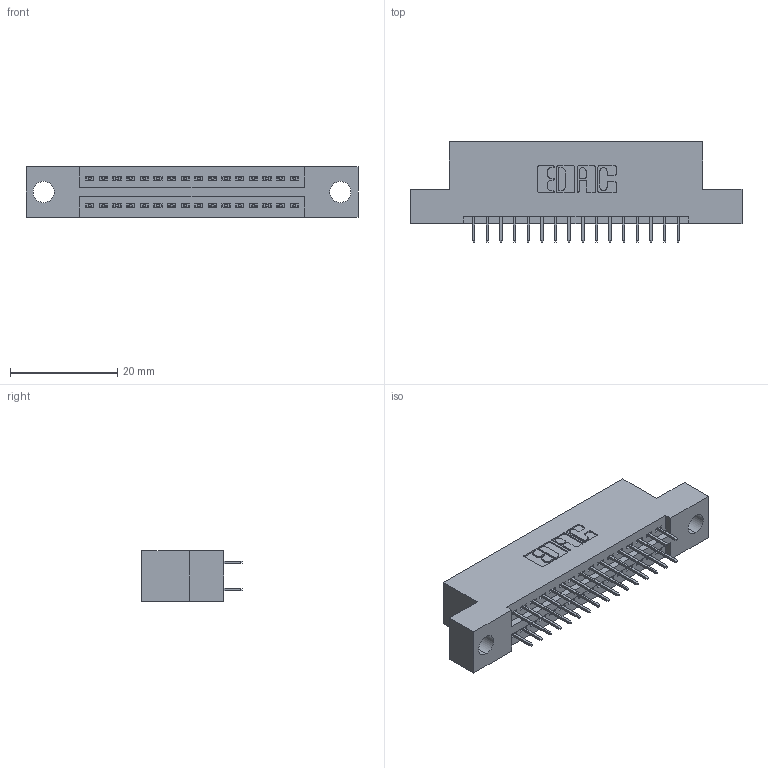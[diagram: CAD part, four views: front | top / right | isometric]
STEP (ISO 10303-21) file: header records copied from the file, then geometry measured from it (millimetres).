
FILE_DESCRIPTION (( 'STEP AP203' ), '1' );
FILE_NAME ('345-032-525-204.STEP', '2020-09-19T13:54:55', ( '' ), ( '' ), 'SwSTEP 2.0', 'SolidWorks 2020', '' );
FILE_SCHEMA (( 'CONFIG_CONTROL_DESIGN' ));
Length unit declared in the file: inch
Products named in the file (3): 345-292-001_345-293-125; 345 Part_Flush Mounting Lugs - 0.156 Dia-TH; 345-032-525-204
Assembly tree (33 placements, depth 2):
  345-032-525-204
    345 Part_Flush Mounting Lugs - 0.156 Dia-TH
    345-292-001_345-293-125  x32
Bounding box: 61.85 x 18.72 x 9.4 mm (x, y, z)
Volume: 5626.2 mm3; surface area: 7469.4 mm2
Topology: 33 solids, 33 shells, 1854 faces, 5237 edges, 3362 vertices
Faces by surface type: plane 1328, cylinder 526
Entity records: 16131 total; most frequent: CARTESIAN_POINT 2728, ORIENTED_EDGE 2662, DIRECTION 2439, EDGE_CURVE 1331, VECTOR 1139, LINE 1139, VERTEX_POINT 882, AXIS2_PLACEMENT_3D 650
